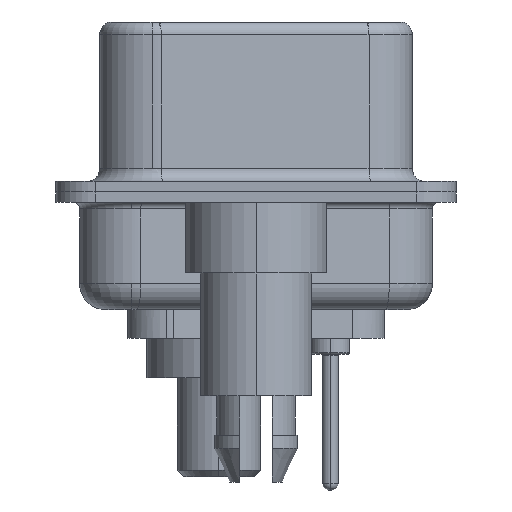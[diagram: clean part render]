
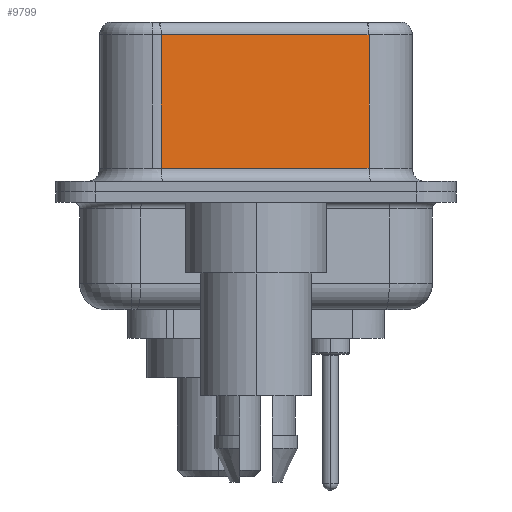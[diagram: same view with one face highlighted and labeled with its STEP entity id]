
A CAD part, left-side view. The second image highlights one B-rep face of the part: STEP entity #9799.
In plain terms, the highlighted planar face has unit normal (-0.985, -0.174, 0).
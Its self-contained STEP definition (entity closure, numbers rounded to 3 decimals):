
#709 = DIRECTION ( 'NONE',  ( 0., 0., -1. ) ) ;
#1229 = CARTESIAN_POINT ( 'NONE',  ( 5.132, -4.322, 0.9 ) ) ;
#1932 = ORIENTED_EDGE ( 'NONE', *, *, #8782, .T. ) ;
#2540 = CARTESIAN_POINT ( 'NONE',  ( 5.132, -4.322, 6.02 ) ) ;
#3076 = ORIENTED_EDGE ( 'NONE', *, *, #16003, .F. ) ;
#5928 = DIRECTION ( 'NONE',  ( 0.985, 0.174, 0. ) ) ;
#6431 = LINE ( 'NONE', #12736, #11176 ) ;
#6474 = AXIS2_PLACEMENT_3D ( 'NONE', #22070, #5928, #20093 ) ;
#7384 = CARTESIAN_POINT ( 'NONE',  ( 3.73, 3.628, 0.9 ) ) ;
#7445 = EDGE_CURVE ( 'NONE', #22126, #11621, #6431, .T. ) ;
#7578 = VERTEX_POINT ( 'NONE', #1229 ) ;
#8190 = ORIENTED_EDGE ( 'NONE', *, *, #10256, .T. ) ;
#8782 = EDGE_CURVE ( 'NONE', #18781, #7578, #10203, .T. ) ;
#9799 = ADVANCED_FACE ( 'NONE', ( #16768 ), #11847, .F. ) ;
#9805 = EDGE_LOOP ( 'NONE', ( #3076, #12375, #8190, #1932 ) ) ;
#10203 = LINE ( 'NONE', #16396, #20364 ) ;
#10256 = EDGE_CURVE ( 'NONE', #11621, #18781, #14555, .T. ) ;
#10429 = DIRECTION ( 'NONE',  ( 0.174, -0.985, 0. ) ) ;
#10823 = CARTESIAN_POINT ( 'NONE',  ( 3.73, 3.628, 6.52 ) ) ;
#10902 = DIRECTION ( 'NONE',  ( -0.174, 0.985, 0. ) ) ;
#11176 = VECTOR ( 'NONE', #10902, 1000. ) ;
#11621 = VERTEX_POINT ( 'NONE', #20239 ) ;
#11847 = PLANE ( 'NONE',  #6474 ) ;
#12375 = ORIENTED_EDGE ( 'NONE', *, *, #7445, .T. ) ;
#12736 = CARTESIAN_POINT ( 'NONE',  ( 5.132, -4.322, 6.02 ) ) ;
#14555 = LINE ( 'NONE', #10823, #19329 ) ;
#15522 = LINE ( 'NONE', #16478, #25114 ) ;
#16003 = EDGE_CURVE ( 'NONE', #22126, #7578, #15522, .T. ) ;
#16396 = CARTESIAN_POINT ( 'NONE',  ( 5.132, -4.322, 0.9 ) ) ;
#16478 = CARTESIAN_POINT ( 'NONE',  ( 5.132, -4.322, 6.52 ) ) ;
#16768 = FACE_OUTER_BOUND ( 'NONE', #9805, .T. ) ;
#18781 = VERTEX_POINT ( 'NONE', #7384 ) ;
#19329 = VECTOR ( 'NONE', #709, 1000. ) ;
#20093 = DIRECTION ( 'NONE',  ( -0.174, 0.985, 0. ) ) ;
#20239 = CARTESIAN_POINT ( 'NONE',  ( 3.73, 3.628, 6.02 ) ) ;
#20364 = VECTOR ( 'NONE', #10429, 1000. ) ;
#22070 = CARTESIAN_POINT ( 'NONE',  ( 5.132, -4.322, 6.52 ) ) ;
#22126 = VERTEX_POINT ( 'NONE', #2540 ) ;
#22668 = DIRECTION ( 'NONE',  ( 0., 0., -1. ) ) ;
#25114 = VECTOR ( 'NONE', #22668, 1000. ) ;
